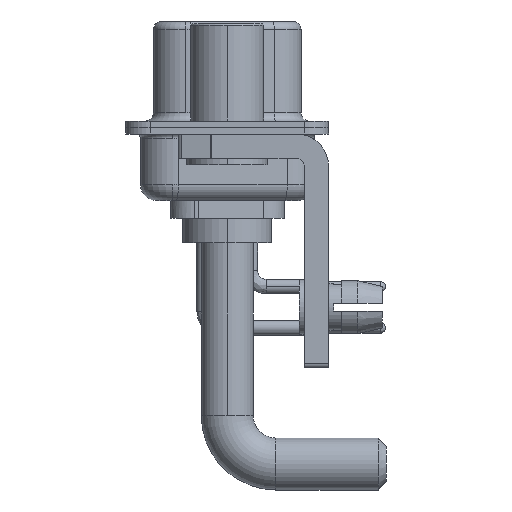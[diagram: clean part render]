
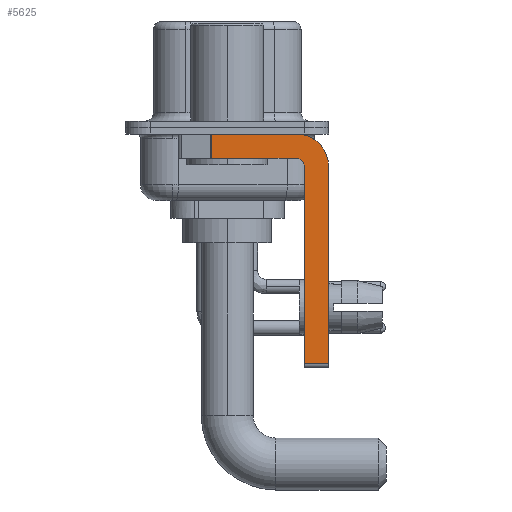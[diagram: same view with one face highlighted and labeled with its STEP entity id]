
A CAD part, left-side view. The second image highlights one B-rep face of the part: STEP entity #5625.
In plain terms, the highlighted planar face has unit normal (-1, 0, 0).
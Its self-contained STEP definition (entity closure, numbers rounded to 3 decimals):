
#378 = CIRCLE ( 'NONE', #2240, 2. ) ;
#1405 = CARTESIAN_POINT ( 'NONE',  ( -2.9, 0.978, -0.4 ) ) ;
#1529 = VECTOR ( 'NONE', #16493, 1000. ) ;
#1775 = ORIENTED_EDGE ( 'NONE', *, *, #24564, .F. ) ;
#1826 = CARTESIAN_POINT ( 'NONE',  ( -2.9, 3., -0.4 ) ) ;
#2145 = ORIENTED_EDGE ( 'NONE', *, *, #16419, .T. ) ;
#2240 = AXIS2_PLACEMENT_3D ( 'NONE', #16437, #3156, #18479 ) ;
#2338 = LINE ( 'NONE', #26620, #7586 ) ;
#2560 = DIRECTION ( 'NONE',  ( 0., 0., 1. ) ) ;
#3156 = DIRECTION ( 'NONE',  ( 1., 0., 0. ) ) ;
#3287 = DIRECTION ( 'NONE',  ( 0., 0., 1. ) ) ;
#3682 = EDGE_CURVE ( 'NONE', #21320, #13362, #28598, .T. ) ;
#4088 = ORIENTED_EDGE ( 'NONE', *, *, #6141, .F. ) ;
#4456 = AXIS2_PLACEMENT_3D ( 'NONE', #14276, #23110, #3287 ) ;
#4728 = VERTEX_POINT ( 'NONE', #27873 ) ;
#4953 = PLANE ( 'NONE',  #16278 ) ;
#5625 = ADVANCED_FACE ( 'NONE', ( #18099 ), #4953, .F. ) ;
#5841 = EDGE_CURVE ( 'NONE', #14704, #7581, #2338, .T. ) ;
#6141 = EDGE_CURVE ( 'NONE', #26751, #4728, #27626, .T. ) ;
#6691 = CARTESIAN_POINT ( 'NONE',  ( -2.9, -4.75, -14.55 ) ) ;
#7185 = LINE ( 'NONE', #20187, #25459 ) ;
#7440 = ORIENTED_EDGE ( 'NONE', *, *, #5841, .F. ) ;
#7522 = CARTESIAN_POINT ( 'NONE',  ( -2.9, -4.25, -1.9 ) ) ;
#7581 = VERTEX_POINT ( 'NONE', #12418 ) ;
#7586 = VECTOR ( 'NONE', #8405, 1000. ) ;
#8121 = DIRECTION ( 'NONE',  ( 0., -1., 0. ) ) ;
#8260 = DIRECTION ( 'NONE',  ( 1., 0., 0. ) ) ;
#8405 = DIRECTION ( 'NONE',  ( 0., 0., -1. ) ) ;
#8609 = CIRCLE ( 'NONE', #4456, 0.5 ) ;
#8612 = DIRECTION ( 'NONE',  ( 0., -1., 0. ) ) ;
#10247 = DIRECTION ( 'NONE',  ( 0., 1., 0. ) ) ;
#10453 = CARTESIAN_POINT ( 'NONE',  ( -2.9, -4.75, -2.4 ) ) ;
#10973 = VERTEX_POINT ( 'NONE', #10453 ) ;
#12257 = ORIENTED_EDGE ( 'NONE', *, *, #22646, .F. ) ;
#12418 = CARTESIAN_POINT ( 'NONE',  ( -2.9, -6.25, -14.55 ) ) ;
#13362 = VERTEX_POINT ( 'NONE', #21934 ) ;
#14276 = CARTESIAN_POINT ( 'NONE',  ( -2.9, -4.25, -2.4 ) ) ;
#14503 = EDGE_LOOP ( 'NONE', ( #18727, #2145, #4088, #12257, #19051, #26545, #7440, #1775 ) ) ;
#14537 = VERTEX_POINT ( 'NONE', #6691 ) ;
#14617 = LINE ( 'NONE', #23445, #25021 ) ;
#14704 = VERTEX_POINT ( 'NONE', #25892 ) ;
#15395 = EDGE_CURVE ( 'NONE', #14537, #7581, #14617, .T. ) ;
#16278 = AXIS2_PLACEMENT_3D ( 'NONE', #27944, #8260, #16772 ) ;
#16419 = EDGE_CURVE ( 'NONE', #21320, #4728, #27533, .T. ) ;
#16437 = CARTESIAN_POINT ( 'NONE',  ( -2.9, -4.25, -2.4 ) ) ;
#16493 = DIRECTION ( 'NONE',  ( 0., 0., -1. ) ) ;
#16772 = DIRECTION ( 'NONE',  ( 0., 0., -1. ) ) ;
#18099 = FACE_OUTER_BOUND ( 'NONE', #14503, .T. ) ;
#18479 = DIRECTION ( 'NONE',  ( 0., 0., -1. ) ) ;
#18727 = ORIENTED_EDGE ( 'NONE', *, *, #3682, .F. ) ;
#19051 = ORIENTED_EDGE ( 'NONE', *, *, #28531, .F. ) ;
#20187 = CARTESIAN_POINT ( 'NONE',  ( -2.9, -4.75, -14.8 ) ) ;
#20426 = CARTESIAN_POINT ( 'NONE',  ( -2.9, 0.978, -1.9 ) ) ;
#20694 = VECTOR ( 'NONE', #8612, 1000. ) ;
#21320 = VERTEX_POINT ( 'NONE', #1405 ) ;
#21889 = VECTOR ( 'NONE', #10247, 1000. ) ;
#21934 = CARTESIAN_POINT ( 'NONE',  ( -2.9, -4.25, -0.4 ) ) ;
#22646 = EDGE_CURVE ( 'NONE', #10973, #26751, #8609, .T. ) ;
#23110 = DIRECTION ( 'NONE',  ( -1., 0., 0. ) ) ;
#23445 = CARTESIAN_POINT ( 'NONE',  ( -2.9, -4.25, -14.55 ) ) ;
#24564 = EDGE_CURVE ( 'NONE', #13362, #14704, #378, .T. ) ;
#25021 = VECTOR ( 'NONE', #8121, 1000. ) ;
#25459 = VECTOR ( 'NONE', #2560, 1000. ) ;
#25833 = CARTESIAN_POINT ( 'NONE',  ( -2.9, -4.25, -1.9 ) ) ;
#25892 = CARTESIAN_POINT ( 'NONE',  ( -2.9, -6.25, -2.4 ) ) ;
#26545 = ORIENTED_EDGE ( 'NONE', *, *, #15395, .T. ) ;
#26620 = CARTESIAN_POINT ( 'NONE',  ( -2.9, -6.25, -2.4 ) ) ;
#26751 = VERTEX_POINT ( 'NONE', #25833 ) ;
#27533 = LINE ( 'NONE', #20426, #1529 ) ;
#27626 = LINE ( 'NONE', #7522, #21889 ) ;
#27873 = CARTESIAN_POINT ( 'NONE',  ( -2.9, 0.978, -1.9 ) ) ;
#27944 = CARTESIAN_POINT ( 'NONE',  ( -2.9, -4.25, -2.4 ) ) ;
#28531 = EDGE_CURVE ( 'NONE', #14537, #10973, #7185, .T. ) ;
#28598 = LINE ( 'NONE', #1826, #20694 ) ;
